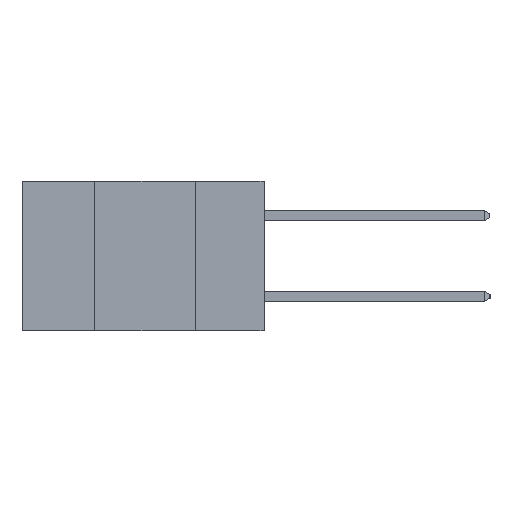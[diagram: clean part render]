
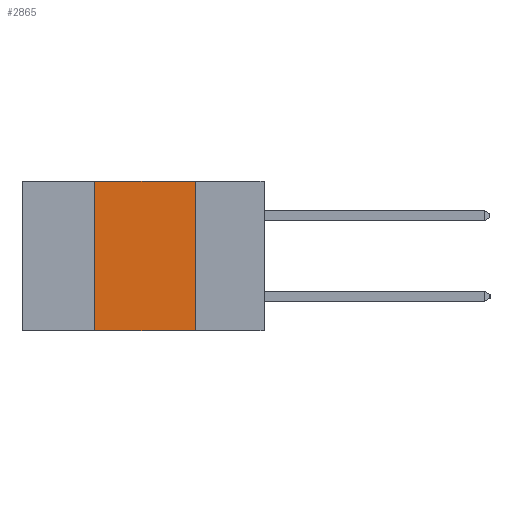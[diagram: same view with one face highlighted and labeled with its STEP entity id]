
A CAD part, left-side view. The second image highlights one B-rep face of the part: STEP entity #2865.
In plain terms, the highlighted planar face has unit normal (-1, 0, 0).
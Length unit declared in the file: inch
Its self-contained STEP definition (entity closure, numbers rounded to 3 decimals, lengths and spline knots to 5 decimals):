
#49 = CARTESIAN_POINT ( 'NONE',  ( 0., 0.42, 0. ) ) ;
#655 = CARTESIAN_POINT ( 'NONE',  ( 0., 0.42, -0.37 ) ) ;
#1339 = DIRECTION ( 'NONE',  ( 0., -1., 0. ) ) ;
#1628 = LINE ( 'NONE', #4354, #10659 ) ;
#1948 = VECTOR ( 'NONE', #5469, 39.37008 ) ;
#1986 = AXIS2_PLACEMENT_3D ( 'NONE', #5610, #6549, #6523 ) ;
#2169 = VERTEX_POINT ( 'NONE', #49 ) ;
#2457 = VERTEX_POINT ( 'NONE', #4722 ) ;
#2865 = ADVANCED_FACE ( 'NONE', ( #9901 ), #4110, .F. ) ;
#2942 = DIRECTION ( 'NONE',  ( 0., 0., 1. ) ) ;
#3157 = VECTOR ( 'NONE', #2942, 39.37008 ) ;
#3410 = DIRECTION ( 'NONE',  ( 0., 0., -1. ) ) ;
#3605 = CARTESIAN_POINT ( 'NONE',  ( 0., 0.6, 0. ) ) ;
#4110 = PLANE ( 'NONE',  #1986 ) ;
#4354 = CARTESIAN_POINT ( 'NONE',  ( 0., 0.17, -0.37 ) ) ;
#4381 = CARTESIAN_POINT ( 'NONE',  ( 0., 0.17, 0. ) ) ;
#4722 = CARTESIAN_POINT ( 'NONE',  ( 0., 0.17, -0.37 ) ) ;
#4754 = LINE ( 'NONE', #3605, #1948 ) ;
#5469 = DIRECTION ( 'NONE',  ( 0., -1., 0. ) ) ;
#5604 = LINE ( 'NONE', #11692, #3157 ) ;
#5610 = CARTESIAN_POINT ( 'NONE',  ( 0., 0.6, 0. ) ) ;
#5968 = VERTEX_POINT ( 'NONE', #4381 ) ;
#6056 = CARTESIAN_POINT ( 'NONE',  ( 0., 0.6, -0.37 ) ) ;
#6351 = EDGE_LOOP ( 'NONE', ( #9157, #11310, #9700, #7344 ) ) ;
#6523 = DIRECTION ( 'NONE',  ( 0., 0., -1. ) ) ;
#6549 = DIRECTION ( 'NONE',  ( 1., 0., 0. ) ) ;
#7344 = ORIENTED_EDGE ( 'NONE', *, *, #8632, .T. ) ;
#8603 = VECTOR ( 'NONE', #1339, 39.37008 ) ;
#8632 = EDGE_CURVE ( 'NONE', #10550, #2457, #9141, .T. ) ;
#9141 = LINE ( 'NONE', #6056, #8603 ) ;
#9157 = ORIENTED_EDGE ( 'NONE', *, *, #10333, .F. ) ;
#9213 = EDGE_CURVE ( 'NONE', #10550, #2169, #5604, .T. ) ;
#9700 = ORIENTED_EDGE ( 'NONE', *, *, #9213, .F. ) ;
#9789 = EDGE_CURVE ( 'NONE', #2169, #5968, #4754, .T. ) ;
#9901 = FACE_OUTER_BOUND ( 'NONE', #6351, .T. ) ;
#10333 = EDGE_CURVE ( 'NONE', #5968, #2457, #1628, .T. ) ;
#10550 = VERTEX_POINT ( 'NONE', #655 ) ;
#10659 = VECTOR ( 'NONE', #3410, 39.37008 ) ;
#11310 = ORIENTED_EDGE ( 'NONE', *, *, #9789, .F. ) ;
#11692 = CARTESIAN_POINT ( 'NONE',  ( 0., 0.42, -0.37 ) ) ;
